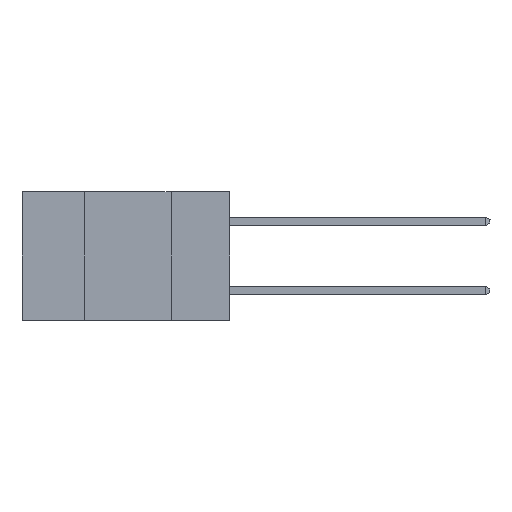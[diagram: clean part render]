
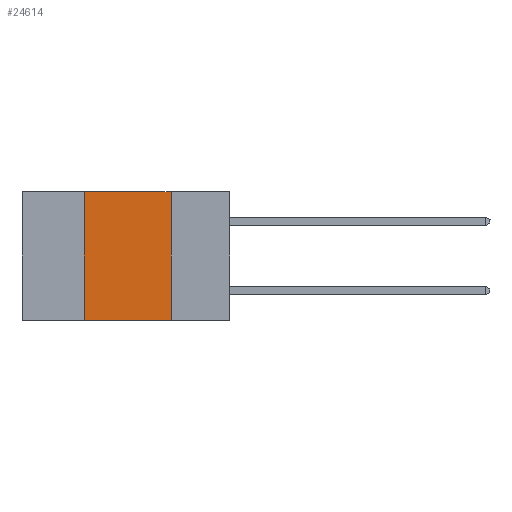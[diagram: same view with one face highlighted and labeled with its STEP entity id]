
A CAD part, left-side view. The second image highlights one B-rep face of the part: STEP entity #24614.
In plain terms, the highlighted planar face has unit normal (-1, 0, 0).
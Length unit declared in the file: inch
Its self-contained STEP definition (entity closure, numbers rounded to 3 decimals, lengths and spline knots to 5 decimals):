
#630 = DIRECTION ( 'NONE',  ( 0., 0., -1. ) ) ;
#1638 = DIRECTION ( 'NONE',  ( 1., 0., 0. ) ) ;
#1973 = DIRECTION ( 'NONE',  ( 0., -1., 0. ) ) ;
#7475 = VECTOR ( 'NONE', #15775, 39.37008 ) ;
#8467 = VECTOR ( 'NONE', #20226, 39.37008 ) ;
#9823 = ORIENTED_EDGE ( 'NONE', *, *, #21226, .F. ) ;
#10968 = EDGE_LOOP ( 'NONE', ( #12920, #9823, #15417, #15305 ) ) ;
#12920 = ORIENTED_EDGE ( 'NONE', *, *, #13341, .F. ) ;
#13341 = EDGE_CURVE ( 'NONE', #21315, #20008, #23605, .T. ) ;
#13391 = VECTOR ( 'NONE', #630, 39.37008 ) ;
#13661 = LINE ( 'NONE', #13671, #7475 ) ;
#13671 = CARTESIAN_POINT ( 'NONE',  ( 0., 0.42, 0. ) ) ;
#14284 = CARTESIAN_POINT ( 'NONE',  ( 0., 0.42, 0. ) ) ;
#14288 = CARTESIAN_POINT ( 'NONE',  ( 0., 0.6, 0. ) ) ;
#15305 = ORIENTED_EDGE ( 'NONE', *, *, #17016, .T. ) ;
#15417 = ORIENTED_EDGE ( 'NONE', *, *, #21594, .F. ) ;
#15775 = DIRECTION ( 'NONE',  ( 0., 0., 1. ) ) ;
#16389 = DIRECTION ( 'NONE',  ( 0., 0., -1. ) ) ;
#17016 = EDGE_CURVE ( 'NONE', #26278, #20008, #19467, .T. ) ;
#17094 = VERTEX_POINT ( 'NONE', #14284 ) ;
#18150 = FACE_OUTER_BOUND ( 'NONE', #10968, .T. ) ;
#18755 = CARTESIAN_POINT ( 'NONE',  ( 0., 0.17, -0.37 ) ) ;
#19467 = LINE ( 'NONE', #24166, #8467 ) ;
#19560 = AXIS2_PLACEMENT_3D ( 'NONE', #14288, #1638, #16389 ) ;
#20008 = VERTEX_POINT ( 'NONE', #18755 ) ;
#20226 = DIRECTION ( 'NONE',  ( 0., -1., 0. ) ) ;
#21226 = EDGE_CURVE ( 'NONE', #17094, #21315, #22660, .T. ) ;
#21315 = VERTEX_POINT ( 'NONE', #25059 ) ;
#21594 = EDGE_CURVE ( 'NONE', #26278, #17094, #13661, .T. ) ;
#22040 = VECTOR ( 'NONE', #1973, 39.37008 ) ;
#22660 = LINE ( 'NONE', #24818, #22040 ) ;
#23605 = LINE ( 'NONE', #25483, #13391 ) ;
#24166 = CARTESIAN_POINT ( 'NONE',  ( 0., 0.6, -0.37 ) ) ;
#24614 = ADVANCED_FACE ( 'NONE', ( #18150 ), #26409, .F. ) ;
#24818 = CARTESIAN_POINT ( 'NONE',  ( 0., 0.6, 0. ) ) ;
#25059 = CARTESIAN_POINT ( 'NONE',  ( 0., 0.17, 0. ) ) ;
#25483 = CARTESIAN_POINT ( 'NONE',  ( 0., 0.17, 0. ) ) ;
#25830 = CARTESIAN_POINT ( 'NONE',  ( 0., 0.42, -0.37 ) ) ;
#26278 = VERTEX_POINT ( 'NONE', #25830 ) ;
#26409 = PLANE ( 'NONE',  #19560 ) ;
